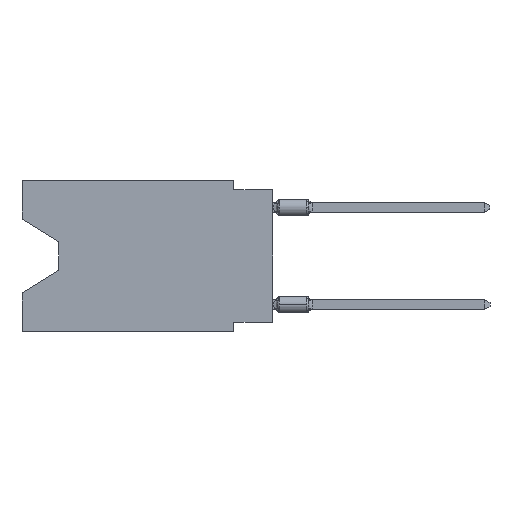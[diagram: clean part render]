
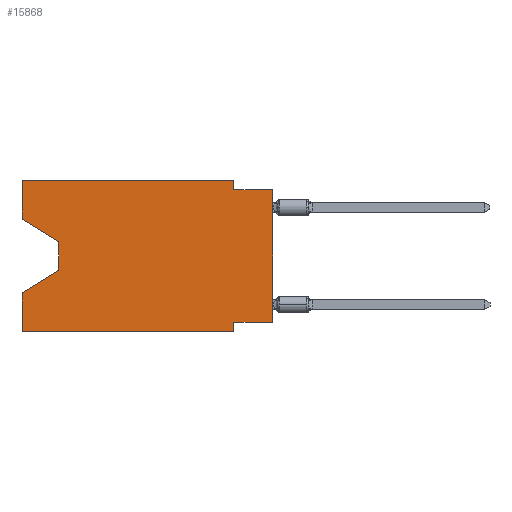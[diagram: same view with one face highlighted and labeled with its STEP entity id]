
A CAD part, left-side view. The second image highlights one B-rep face of the part: STEP entity #15868.
In plain terms, the highlighted planar face has unit normal (-1, 0, 0).
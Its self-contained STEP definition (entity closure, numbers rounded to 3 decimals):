
#357 = EDGE_CURVE ( 'NONE', #15236, #10864, #6466, .T. ) ;
#459 = EDGE_CURVE ( 'NONE', #19485, #2006, #16441, .T. ) ;
#689 = LINE ( 'NONE', #20484, #3523 ) ;
#823 = LINE ( 'NONE', #5701, #20645 ) ;
#1237 = VERTEX_POINT ( 'NONE', #21255 ) ;
#1652 = LINE ( 'NONE', #4896, #15733 ) ;
#1700 = ORIENTED_EDGE ( 'NONE', *, *, #6308, .F. ) ;
#1800 = ORIENTED_EDGE ( 'NONE', *, *, #2166, .T. ) ;
#2006 = VERTEX_POINT ( 'NONE', #5764 ) ;
#2164 = EDGE_CURVE ( 'NONE', #15236, #10926, #11783, .T. ) ;
#2166 = EDGE_CURVE ( 'NONE', #10926, #9589, #12167, .T. ) ;
#2258 = VECTOR ( 'NONE', #10044, 1000. ) ;
#2438 = EDGE_CURVE ( 'NONE', #3491, #12578, #20496, .T. ) ;
#2780 = CARTESIAN_POINT ( 'NONE',  ( 0., 16.383, 0. ) ) ;
#2858 = EDGE_LOOP ( 'NONE', ( #4029, #1800, #19626, #5693, #13821, #16296, #11025, #14045, #1700, #13283, #11726, #8214 ) ) ;
#3349 = VECTOR ( 'NONE', #16220, 1000. ) ;
#3473 = VERTEX_POINT ( 'NONE', #8421 ) ;
#3491 = VERTEX_POINT ( 'NONE', #11771 ) ;
#3523 = VECTOR ( 'NONE', #9107, 1000. ) ;
#3605 = DIRECTION ( 'NONE',  ( 0., 0.855, -0.519 ) ) ;
#4029 = ORIENTED_EDGE ( 'NONE', *, *, #2164, .T. ) ;
#4034 = CARTESIAN_POINT ( 'NONE',  ( 0., 13.97, -4.013 ) ) ;
#4075 = EDGE_CURVE ( 'NONE', #9589, #12578, #6861, .T. ) ;
#4896 = CARTESIAN_POINT ( 'NONE',  ( 0., 16.383, -9.906 ) ) ;
#4929 = DIRECTION ( 'NONE',  ( 0., 0., -1. ) ) ;
#5420 = CARTESIAN_POINT ( 'NONE',  ( 0., 13.97, -4.013 ) ) ;
#5693 = ORIENTED_EDGE ( 'NONE', *, *, #2438, .F. ) ;
#5701 = CARTESIAN_POINT ( 'NONE',  ( 0., 16.383, 0. ) ) ;
#5764 = CARTESIAN_POINT ( 'NONE',  ( 0., 2.54, -9.906 ) ) ;
#6308 = EDGE_CURVE ( 'NONE', #3473, #1237, #9673, .T. ) ;
#6466 = LINE ( 'NONE', #2780, #19578 ) ;
#6856 = CARTESIAN_POINT ( 'NONE',  ( 0., 2.54, -9.271 ) ) ;
#6861 = LINE ( 'NONE', #13438, #13156 ) ;
#7236 = DIRECTION ( 'NONE',  ( 1., 0., 0. ) ) ;
#7298 = DIRECTION ( 'NONE',  ( 0., 0., 1. ) ) ;
#7842 = VECTOR ( 'NONE', #15253, 1000. ) ;
#8090 = EDGE_CURVE ( 'NONE', #16459, #3473, #8481, .T. ) ;
#8109 = CARTESIAN_POINT ( 'NONE',  ( 0., 13.97, -5.893 ) ) ;
#8214 = ORIENTED_EDGE ( 'NONE', *, *, #357, .F. ) ;
#8421 = CARTESIAN_POINT ( 'NONE',  ( 0., 2.54, -0.635 ) ) ;
#8481 = LINE ( 'NONE', #16389, #19232 ) ;
#8580 = EDGE_CURVE ( 'NONE', #10864, #16459, #823, .T. ) ;
#8900 = VERTEX_POINT ( 'NONE', #13345 ) ;
#9107 = DIRECTION ( 'NONE',  ( 0., 0., 1. ) ) ;
#9253 = DIRECTION ( 'NONE',  ( 0., 0., 1. ) ) ;
#9589 = VERTEX_POINT ( 'NONE', #8109 ) ;
#9673 = LINE ( 'NONE', #19871, #11325 ) ;
#9838 = VECTOR ( 'NONE', #7298, 1000. ) ;
#10041 = EDGE_CURVE ( 'NONE', #8900, #1237, #689, .T. ) ;
#10044 = DIRECTION ( 'NONE',  ( 0., 0., -1. ) ) ;
#10152 = DIRECTION ( 'NONE',  ( 0., -0.855, -0.519 ) ) ;
#10578 = CARTESIAN_POINT ( 'NONE',  ( 0., 16.383, 0. ) ) ;
#10714 = LINE ( 'NONE', #17008, #7842 ) ;
#10864 = VERTEX_POINT ( 'NONE', #11680 ) ;
#10926 = VERTEX_POINT ( 'NONE', #5420 ) ;
#11025 = ORIENTED_EDGE ( 'NONE', *, *, #20692, .F. ) ;
#11325 = VECTOR ( 'NONE', #16410, 1000. ) ;
#11477 = DIRECTION ( 'NONE',  ( 0., -1., 0. ) ) ;
#11565 = CARTESIAN_POINT ( 'NONE',  ( 0., 16.383, -2.546 ) ) ;
#11680 = CARTESIAN_POINT ( 'NONE',  ( 0., 16.383, 0. ) ) ;
#11726 = ORIENTED_EDGE ( 'NONE', *, *, #8580, .F. ) ;
#11771 = CARTESIAN_POINT ( 'NONE',  ( 0., 16.383, -9.906 ) ) ;
#11783 = LINE ( 'NONE', #11565, #18154 ) ;
#12060 = DIRECTION ( 'NONE',  ( 0., -1., 0. ) ) ;
#12167 = LINE ( 'NONE', #4034, #2258 ) ;
#12168 = CARTESIAN_POINT ( 'NONE',  ( 0., 2.54, 0. ) ) ;
#12373 = CARTESIAN_POINT ( 'NONE',  ( 0., 16.383, 0. ) ) ;
#12578 = VERTEX_POINT ( 'NONE', #19685 ) ;
#13156 = VECTOR ( 'NONE', #3605, 1000. ) ;
#13283 = ORIENTED_EDGE ( 'NONE', *, *, #8090, .F. ) ;
#13345 = CARTESIAN_POINT ( 'NONE',  ( 0., 0., -9.271 ) ) ;
#13438 = CARTESIAN_POINT ( 'NONE',  ( 0., 13.97, -5.893 ) ) ;
#13450 = EDGE_CURVE ( 'NONE', #3491, #2006, #1652, .T. ) ;
#13810 = DIRECTION ( 'NONE',  ( 0., 0., -1. ) ) ;
#13821 = ORIENTED_EDGE ( 'NONE', *, *, #13450, .T. ) ;
#13869 = AXIS2_PLACEMENT_3D ( 'NONE', #10578, #7236, #13810 ) ;
#14045 = ORIENTED_EDGE ( 'NONE', *, *, #10041, .T. ) ;
#15236 = VERTEX_POINT ( 'NONE', #15979 ) ;
#15253 = DIRECTION ( 'NONE',  ( 0., 1., 0. ) ) ;
#15733 = VECTOR ( 'NONE', #11477, 1000. ) ;
#15868 = ADVANCED_FACE ( 'NONE', ( #20017 ), #17198, .F. ) ;
#15979 = CARTESIAN_POINT ( 'NONE',  ( 0., 16.383, -2.546 ) ) ;
#16220 = DIRECTION ( 'NONE',  ( 0., 0., -1. ) ) ;
#16296 = ORIENTED_EDGE ( 'NONE', *, *, #459, .F. ) ;
#16389 = CARTESIAN_POINT ( 'NONE',  ( 0., 2.54, 0. ) ) ;
#16410 = DIRECTION ( 'NONE',  ( 0., -1., 0. ) ) ;
#16441 = LINE ( 'NONE', #18168, #3349 ) ;
#16459 = VERTEX_POINT ( 'NONE', #12168 ) ;
#17008 = CARTESIAN_POINT ( 'NONE',  ( 0., 0., -9.271 ) ) ;
#17198 = PLANE ( 'NONE',  #13869 ) ;
#18154 = VECTOR ( 'NONE', #10152, 1000. ) ;
#18168 = CARTESIAN_POINT ( 'NONE',  ( 0., 2.54, -9.906 ) ) ;
#19232 = VECTOR ( 'NONE', #4929, 1000. ) ;
#19485 = VERTEX_POINT ( 'NONE', #6856 ) ;
#19578 = VECTOR ( 'NONE', #9253, 1000. ) ;
#19626 = ORIENTED_EDGE ( 'NONE', *, *, #4075, .T. ) ;
#19685 = CARTESIAN_POINT ( 'NONE',  ( 0., 16.383, -7.36 ) ) ;
#19871 = CARTESIAN_POINT ( 'NONE',  ( 0., 0., -0.635 ) ) ;
#20017 = FACE_OUTER_BOUND ( 'NONE', #2858, .T. ) ;
#20484 = CARTESIAN_POINT ( 'NONE',  ( 0., 0., 0. ) ) ;
#20496 = LINE ( 'NONE', #12373, #9838 ) ;
#20645 = VECTOR ( 'NONE', #12060, 1000. ) ;
#20692 = EDGE_CURVE ( 'NONE', #8900, #19485, #10714, .T. ) ;
#21255 = CARTESIAN_POINT ( 'NONE',  ( 0., 0., -0.635 ) ) ;
